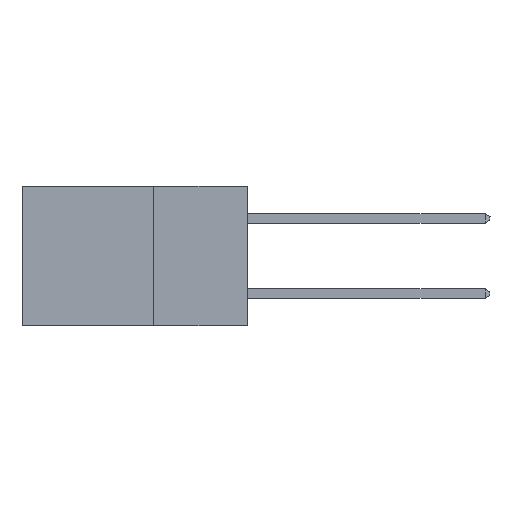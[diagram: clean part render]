
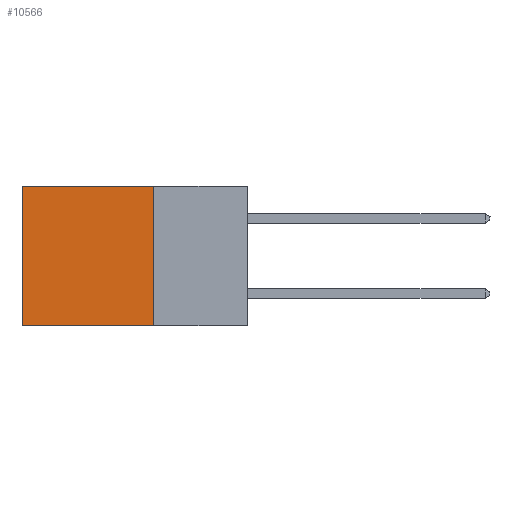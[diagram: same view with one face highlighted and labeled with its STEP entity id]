
A CAD part, left-side view. The second image highlights one B-rep face of the part: STEP entity #10566.
In plain terms, the highlighted planar face has unit normal (-1, 0, 0).
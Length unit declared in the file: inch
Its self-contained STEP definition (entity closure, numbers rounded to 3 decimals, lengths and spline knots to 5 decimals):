
#565 = CARTESIAN_POINT ( 'NONE',  ( 0.2615, 0.25, -0.37 ) ) ;
#1026 = VECTOR ( 'NONE', #4172, 39.37008 ) ;
#1694 = CARTESIAN_POINT ( 'NONE',  ( 0.2615, 0.25, -0.37 ) ) ;
#1743 = EDGE_CURVE ( 'NONE', #9705, #9445, #11473, .T. ) ;
#2243 = DIRECTION ( 'NONE',  ( 0., 1., 0. ) ) ;
#2263 = CARTESIAN_POINT ( 'NONE',  ( 0.2615, 0.25, 0. ) ) ;
#2302 = CARTESIAN_POINT ( 'NONE',  ( 0.2615, 0.25, 0. ) ) ;
#2648 = DIRECTION ( 'NONE',  ( 0., 0., -1. ) ) ;
#2923 = VECTOR ( 'NONE', #2243, 39.37008 ) ;
#3398 = CARTESIAN_POINT ( 'NONE',  ( 0.2615, 0.25, -0.37 ) ) ;
#3568 = EDGE_CURVE ( 'NONE', #9705, #8277, #10301, .T. ) ;
#3585 = LINE ( 'NONE', #7862, #8616 ) ;
#3730 = CARTESIAN_POINT ( 'NONE',  ( 0.2615, 0.25, -0.37 ) ) ;
#4078 = VECTOR ( 'NONE', #10913, 39.37008 ) ;
#4172 = DIRECTION ( 'NONE',  ( 0., 0., -1. ) ) ;
#4365 = VERTEX_POINT ( 'NONE', #8612 ) ;
#4559 = CARTESIAN_POINT ( 'NONE',  ( 0.2615, 0.6, 0. ) ) ;
#4823 = DIRECTION ( 'NONE',  ( 1., 0., 0. ) ) ;
#4884 = PLANE ( 'NONE',  #10146 ) ;
#5942 = ORIENTED_EDGE ( 'NONE', *, *, #1743, .F. ) ;
#6667 = EDGE_CURVE ( 'NONE', #8277, #4365, #3585, .T. ) ;
#7862 = CARTESIAN_POINT ( 'NONE',  ( 0.2615, 0.6, -0.37 ) ) ;
#8127 = LINE ( 'NONE', #3730, #4078 ) ;
#8277 = VERTEX_POINT ( 'NONE', #4559 ) ;
#8606 = EDGE_LOOP ( 'NONE', ( #9574, #9604, #5942, #9678 ) ) ;
#8612 = CARTESIAN_POINT ( 'NONE',  ( 0.2615, 0.6, -0.37 ) ) ;
#8616 = VECTOR ( 'NONE', #2648, 39.37008 ) ;
#9445 = VERTEX_POINT ( 'NONE', #1694 ) ;
#9574 = ORIENTED_EDGE ( 'NONE', *, *, #6667, .T. ) ;
#9604 = ORIENTED_EDGE ( 'NONE', *, *, #10037, .F. ) ;
#9678 = ORIENTED_EDGE ( 'NONE', *, *, #3568, .T. ) ;
#9705 = VERTEX_POINT ( 'NONE', #2263 ) ;
#10037 = EDGE_CURVE ( 'NONE', #9445, #4365, #8127, .T. ) ;
#10065 = FACE_OUTER_BOUND ( 'NONE', #8606, .T. ) ;
#10127 = DIRECTION ( 'NONE',  ( 0., 0., -1. ) ) ;
#10146 = AXIS2_PLACEMENT_3D ( 'NONE', #565, #4823, #10127 ) ;
#10301 = LINE ( 'NONE', #2302, #2923 ) ;
#10566 = ADVANCED_FACE ( 'NONE', ( #10065 ), #4884, .F. ) ;
#10913 = DIRECTION ( 'NONE',  ( 0., 1., 0. ) ) ;
#11473 = LINE ( 'NONE', #3398, #1026 ) ;
